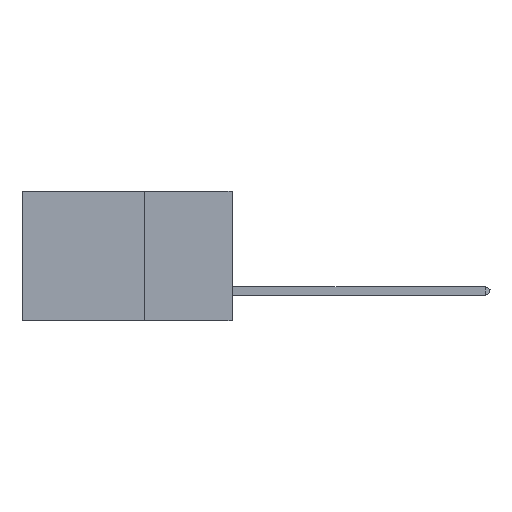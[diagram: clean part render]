
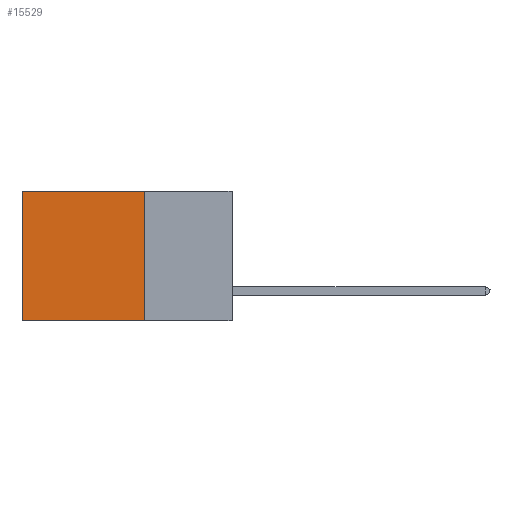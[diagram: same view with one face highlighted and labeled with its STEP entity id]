
A CAD part, left-side view. The second image highlights one B-rep face of the part: STEP entity #15529.
In plain terms, the highlighted planar face has unit normal (-1, 0, 0).
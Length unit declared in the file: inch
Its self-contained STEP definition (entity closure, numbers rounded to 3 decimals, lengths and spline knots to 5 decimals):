
#137 = VECTOR ( 'NONE', #40654, 39.37008 ) ;
#2240 = VERTEX_POINT ( 'NONE', #29591 ) ;
#4460 = ORIENTED_EDGE ( 'NONE', *, *, #24688, .T. ) ;
#4988 = CARTESIAN_POINT ( 'NONE',  ( 0.2875, 0.25, -0.37 ) ) ;
#6727 = AXIS2_PLACEMENT_3D ( 'NONE', #6884, #17302, #20522 ) ;
#6884 = CARTESIAN_POINT ( 'NONE',  ( 0.2875, 0.25, 0. ) ) ;
#7058 = CARTESIAN_POINT ( 'NONE',  ( 0.2875, 0.25, 0. ) ) ;
#7379 = VERTEX_POINT ( 'NONE', #8334 ) ;
#8334 = CARTESIAN_POINT ( 'NONE',  ( 0.2875, 0.6, -0.37 ) ) ;
#10925 = VECTOR ( 'NONE', #18233, 39.37008 ) ;
#11399 = ORIENTED_EDGE ( 'NONE', *, *, #31780, .F. ) ;
#14619 = CARTESIAN_POINT ( 'NONE',  ( 0.2875, 0.25, 0. ) ) ;
#15351 = LINE ( 'NONE', #25318, #22879 ) ;
#15529 = ADVANCED_FACE ( 'NONE', ( #31651 ), #29389, .F. ) ;
#17302 = DIRECTION ( 'NONE',  ( 1., 0., 0. ) ) ;
#17412 = LINE ( 'NONE', #4988, #137 ) ;
#17840 = VERTEX_POINT ( 'NONE', #40449 ) ;
#18233 = DIRECTION ( 'NONE',  ( 0., 1., 0. ) ) ;
#19142 = ORIENTED_EDGE ( 'NONE', *, *, #23019, .T. ) ;
#20522 = DIRECTION ( 'NONE',  ( 0., 0., -1. ) ) ;
#21437 = CARTESIAN_POINT ( 'NONE',  ( 0.2875, 0.25, 0. ) ) ;
#22879 = VECTOR ( 'NONE', #41544, 39.37008 ) ;
#23019 = EDGE_CURVE ( 'NONE', #36552, #17840, #26094, .T. ) ;
#24688 = EDGE_CURVE ( 'NONE', #17840, #7379, #15351, .T. ) ;
#25318 = CARTESIAN_POINT ( 'NONE',  ( 0.2875, 0.6, 0. ) ) ;
#25769 = VECTOR ( 'NONE', #32939, 39.37008 ) ;
#26094 = LINE ( 'NONE', #21437, #10925 ) ;
#29070 = ORIENTED_EDGE ( 'NONE', *, *, #30305, .F. ) ;
#29389 = PLANE ( 'NONE',  #6727 ) ;
#29591 = CARTESIAN_POINT ( 'NONE',  ( 0.2875, 0.25, -0.37 ) ) ;
#30305 = EDGE_CURVE ( 'NONE', #36552, #2240, #40929, .T. ) ;
#31651 = FACE_OUTER_BOUND ( 'NONE', #36873, .T. ) ;
#31780 = EDGE_CURVE ( 'NONE', #2240, #7379, #17412, .T. ) ;
#32939 = DIRECTION ( 'NONE',  ( 0., 0., -1. ) ) ;
#36552 = VERTEX_POINT ( 'NONE', #14619 ) ;
#36873 = EDGE_LOOP ( 'NONE', ( #4460, #11399, #29070, #19142 ) ) ;
#40449 = CARTESIAN_POINT ( 'NONE',  ( 0.2875, 0.6, 0. ) ) ;
#40654 = DIRECTION ( 'NONE',  ( 0., 1., 0. ) ) ;
#40929 = LINE ( 'NONE', #7058, #25769 ) ;
#41544 = DIRECTION ( 'NONE',  ( 0., 0., -1. ) ) ;
